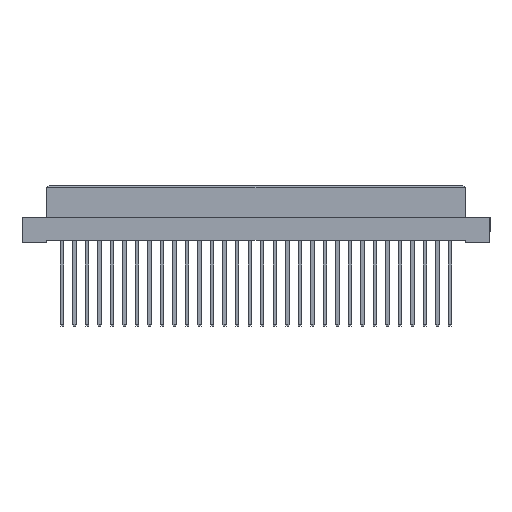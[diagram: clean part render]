
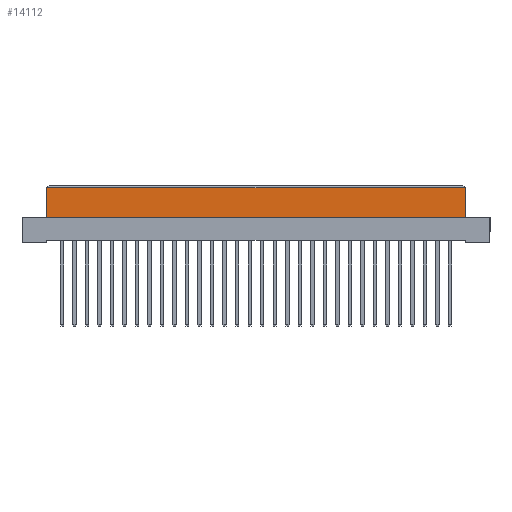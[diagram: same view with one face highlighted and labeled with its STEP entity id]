
A CAD part, top view. The second image highlights one B-rep face of the part: STEP entity #14112.
In plain terms, the highlighted planar face has unit normal (0, 0, 1).
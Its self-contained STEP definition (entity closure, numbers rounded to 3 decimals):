
#54 = LINE ( 'NONE', #3155, #31956 ) ;
#893 = ORIENTED_EDGE ( 'NONE', *, *, #40681, .T. ) ;
#2026 = AXIS2_PLACEMENT_3D ( 'NONE', #8603, #33803, #21607 ) ;
#3155 = CARTESIAN_POINT ( 'NONE',  ( -42.5, -6.4, 4.25 ) ) ;
#3234 = EDGE_CURVE ( 'NONE', #36826, #9426, #27301, .T. ) ;
#8603 = CARTESIAN_POINT ( 'NONE',  ( 42.5, -6.4, 4.25 ) ) ;
#8918 = DIRECTION ( 'NONE',  ( 1., 0., 0. ) ) ;
#9426 = VERTEX_POINT ( 'NONE', #40014 ) ;
#9706 = DIRECTION ( 'NONE',  ( -1., 0., 0. ) ) ;
#10102 = LINE ( 'NONE', #16065, #10780 ) ;
#10194 = ORIENTED_EDGE ( 'NONE', *, *, #3234, .T. ) ;
#10780 = VECTOR ( 'NONE', #31786, 1000. ) ;
#10838 = VECTOR ( 'NONE', #8918, 1000. ) ;
#10850 = CARTESIAN_POINT ( 'NONE',  ( -42.5, -0.5, 4.25 ) ) ;
#11615 = CARTESIAN_POINT ( 'NONE',  ( 42.5, -6.4, 4.25 ) ) ;
#11790 = CARTESIAN_POINT ( 'NONE',  ( -42.5, -0.5, 4.25 ) ) ;
#12648 = DIRECTION ( 'NONE',  ( 0., 1., 0. ) ) ;
#12820 = CARTESIAN_POINT ( 'NONE',  ( -42.5, -6.4, 4.25 ) ) ;
#14112 = ADVANCED_FACE ( 'NONE', ( #18898 ), #18294, .T. ) ;
#16065 = CARTESIAN_POINT ( 'NONE',  ( 42.5, -6.4, 4.25 ) ) ;
#16827 = EDGE_CURVE ( 'NONE', #9426, #34012, #10102, .T. ) ;
#18294 = PLANE ( 'NONE',  #2026 ) ;
#18898 = FACE_OUTER_BOUND ( 'NONE', #34309, .T. ) ;
#19004 = VERTEX_POINT ( 'NONE', #10850 ) ;
#20060 = VECTOR ( 'NONE', #9706, 1000. ) ;
#20576 = EDGE_CURVE ( 'NONE', #36826, #19004, #54, .T. ) ;
#20757 = CARTESIAN_POINT ( 'NONE',  ( 42.5, -0.5, 4.25 ) ) ;
#21607 = DIRECTION ( 'NONE',  ( 1., 0., 0. ) ) ;
#24438 = ORIENTED_EDGE ( 'NONE', *, *, #16827, .T. ) ;
#27301 = LINE ( 'NONE', #11615, #10838 ) ;
#31786 = DIRECTION ( 'NONE',  ( 0., 1., 0. ) ) ;
#31956 = VECTOR ( 'NONE', #12648, 1000. ) ;
#33803 = DIRECTION ( 'NONE',  ( 0., 0., 1. ) ) ;
#34012 = VERTEX_POINT ( 'NONE', #20757 ) ;
#34309 = EDGE_LOOP ( 'NONE', ( #24438, #893, #40546, #10194 ) ) ;
#36826 = VERTEX_POINT ( 'NONE', #12820 ) ;
#40014 = CARTESIAN_POINT ( 'NONE',  ( 42.5, -6.4, 4.25 ) ) ;
#40070 = LINE ( 'NONE', #11790, #20060 ) ;
#40546 = ORIENTED_EDGE ( 'NONE', *, *, #20576, .F. ) ;
#40681 = EDGE_CURVE ( 'NONE', #34012, #19004, #40070, .T. ) ;
